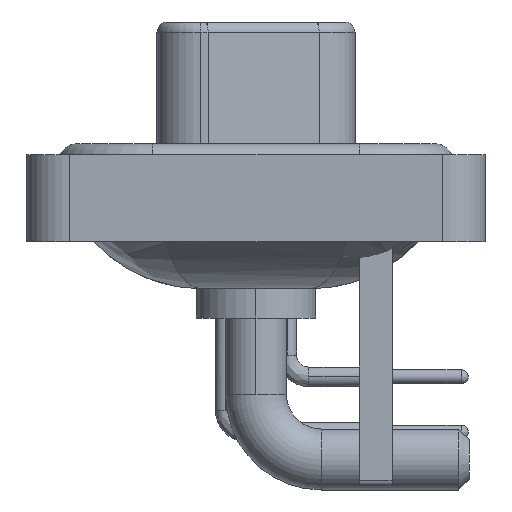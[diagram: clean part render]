
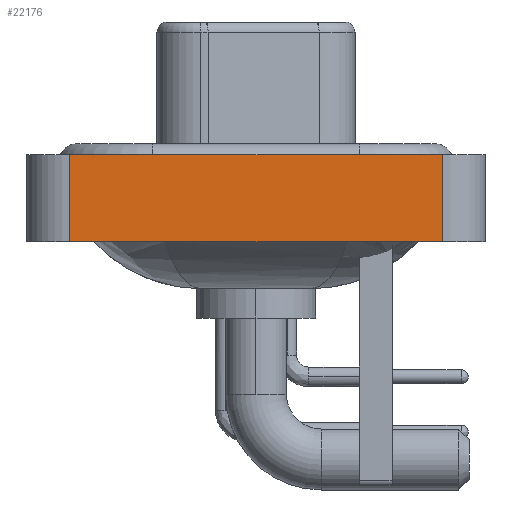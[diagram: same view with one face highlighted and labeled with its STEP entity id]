
A CAD part, left-side view. The second image highlights one B-rep face of the part: STEP entity #22176.
In plain terms, the highlighted planar face has unit normal (-1, 0, 0).
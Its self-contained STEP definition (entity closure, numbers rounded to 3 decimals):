
#94 = ORIENTED_EDGE ( 'NONE', *, *, #1750, .T. ) ;
#173 = CARTESIAN_POINT ( 'NONE',  ( -7.35, -8.55, 0.4 ) ) ;
#347 = DIRECTION ( 'NONE',  ( 0., -1., 0. ) ) ;
#1035 = VECTOR ( 'NONE', #13519, 1000. ) ;
#1245 = CARTESIAN_POINT ( 'NONE',  ( -7.35, -8.55, -3.6 ) ) ;
#1750 = EDGE_CURVE ( 'NONE', #4587, #22790, #26142, .T. ) ;
#2990 = VERTEX_POINT ( 'NONE', #24996 ) ;
#3844 = DIRECTION ( 'NONE',  ( 0., 0., 1. ) ) ;
#4587 = VERTEX_POINT ( 'NONE', #8248 ) ;
#5583 = VECTOR ( 'NONE', #11260, 1000. ) ;
#5604 = EDGE_CURVE ( 'NONE', #22790, #15327, #23065, .T. ) ;
#6204 = EDGE_CURVE ( 'NONE', #4587, #2990, #23980, .T. ) ;
#7912 = DIRECTION ( 'NONE',  ( 0., 0., 1. ) ) ;
#8248 = CARTESIAN_POINT ( 'NONE',  ( -7.35, 8.55, -3.6 ) ) ;
#9399 = CARTESIAN_POINT ( 'NONE',  ( -7.35, 8.55, -3.6 ) ) ;
#11260 = DIRECTION ( 'NONE',  ( 0., -1., 0. ) ) ;
#11545 = LINE ( 'NONE', #15769, #5583 ) ;
#13519 = DIRECTION ( 'NONE',  ( 0., 0., 1. ) ) ;
#14111 = ORIENTED_EDGE ( 'NONE', *, *, #5604, .T. ) ;
#14634 = EDGE_LOOP ( 'NONE', ( #14111, #22996, #24504, #94 ) ) ;
#15327 = VERTEX_POINT ( 'NONE', #173 ) ;
#15769 = CARTESIAN_POINT ( 'NONE',  ( -7.35, -8.55, 0.4 ) ) ;
#17084 = CARTESIAN_POINT ( 'NONE',  ( -7.35, -8.55, -3.6 ) ) ;
#17377 = CARTESIAN_POINT ( 'NONE',  ( -7.35, -8.55, -3.6 ) ) ;
#18739 = CARTESIAN_POINT ( 'NONE',  ( -7.35, -8.55, -3.6 ) ) ;
#22176 = ADVANCED_FACE ( 'NONE', ( #23261 ), #28039, .T. ) ;
#22314 = VECTOR ( 'NONE', #7912, 1000. ) ;
#22790 = VERTEX_POINT ( 'NONE', #17377 ) ;
#22996 = ORIENTED_EDGE ( 'NONE', *, *, #26375, .F. ) ;
#23065 = LINE ( 'NONE', #1245, #22314 ) ;
#23261 = FACE_OUTER_BOUND ( 'NONE', #14634, .T. ) ;
#23980 = LINE ( 'NONE', #9399, #1035 ) ;
#24363 = VECTOR ( 'NONE', #347, 1000. ) ;
#24504 = ORIENTED_EDGE ( 'NONE', *, *, #6204, .F. ) ;
#24996 = CARTESIAN_POINT ( 'NONE',  ( -7.35, 8.55, 0.4 ) ) ;
#25660 = AXIS2_PLACEMENT_3D ( 'NONE', #18739, #25917, #3844 ) ;
#25917 = DIRECTION ( 'NONE',  ( -1., 0., 0. ) ) ;
#26142 = LINE ( 'NONE', #17084, #24363 ) ;
#26375 = EDGE_CURVE ( 'NONE', #2990, #15327, #11545, .T. ) ;
#28039 = PLANE ( 'NONE',  #25660 ) ;
